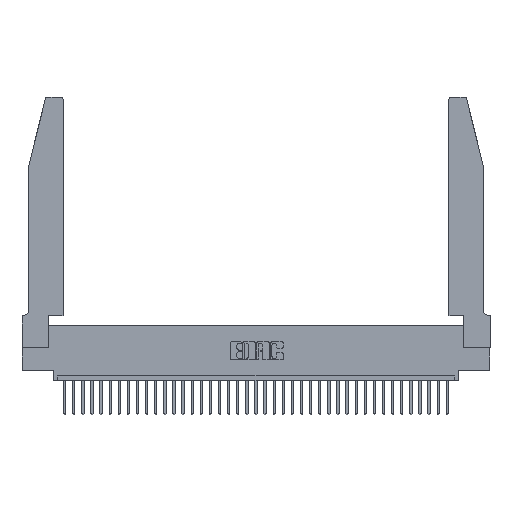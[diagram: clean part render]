
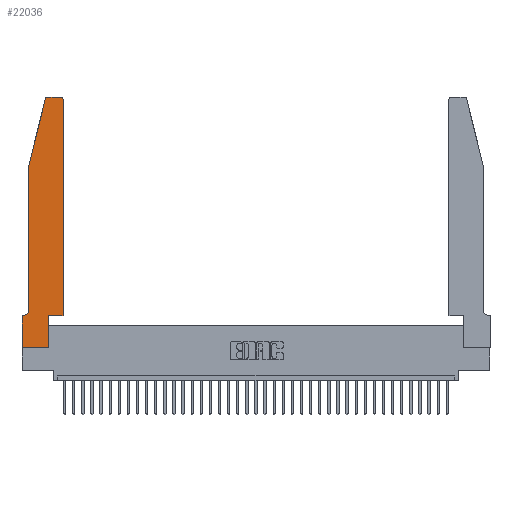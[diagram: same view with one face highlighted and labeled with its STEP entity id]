
A CAD part, top view. The second image highlights one B-rep face of the part: STEP entity #22036.
In plain terms, the highlighted planar face has unit normal (0, 0, 1).
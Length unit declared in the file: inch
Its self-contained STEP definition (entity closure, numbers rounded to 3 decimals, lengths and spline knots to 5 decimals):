
#515 = EDGE_CURVE ( 'NONE', #30148, #27316, #31399, .T. ) ;
#525 = EDGE_CURVE ( 'NONE', #15190, #22995, #31805, .T. ) ;
#536 = DIRECTION ( 'NONE',  ( 0., 0., -1. ) ) ;
#739 = AXIS2_PLACEMENT_3D ( 'NONE', #6330, #9229, #6590 ) ;
#1643 = EDGE_CURVE ( 'NONE', #19819, #7447, #14745, .T. ) ;
#2044 = DIRECTION ( 'NONE',  ( 0., 0., 1. ) ) ;
#2127 = VERTEX_POINT ( 'NONE', #19184 ) ;
#2597 = DIRECTION ( 'NONE',  ( 0., 0., 1. ) ) ;
#2716 = LINE ( 'NONE', #20206, #26402 ) ;
#3038 = DIRECTION ( 'NONE',  ( 0., 1., 0. ) ) ;
#3045 = LINE ( 'NONE', #9687, #5281 ) ;
#3090 = DIRECTION ( 'NONE',  ( -1., 0., 0. ) ) ;
#3216 = CARTESIAN_POINT ( 'NONE',  ( 0.4505, 2.72, 0.37 ) ) ;
#3639 = CARTESIAN_POINT ( 'NONE',  ( 0.0055, 0.35, 0.37 ) ) ;
#5055 = VERTEX_POINT ( 'NONE', #18728 ) ;
#5235 = AXIS2_PLACEMENT_3D ( 'NONE', #31842, #536, #20559 ) ;
#5281 = VECTOR ( 'NONE', #32691, 39.37008 ) ;
#5561 = CARTESIAN_POINT ( 'NONE',  ( 0.0755, 2., 0.37 ) ) ;
#5908 = VERTEX_POINT ( 'NONE', #22934 ) ;
#6234 = VECTOR ( 'NONE', #21673, 39.37008 ) ;
#6330 = CARTESIAN_POINT ( 'NONE',  ( 0.284, 2.72, 0.37 ) ) ;
#6590 = DIRECTION ( 'NONE',  ( 1., 0., 0. ) ) ;
#6735 = ORIENTED_EDGE ( 'NONE', *, *, #24252, .T. ) ;
#7035 = VECTOR ( 'NONE', #9014, 39.37008 ) ;
#7376 = ORIENTED_EDGE ( 'NONE', *, *, #33072, .T. ) ;
#7447 = VERTEX_POINT ( 'NONE', #3216 ) ;
#8647 = ORIENTED_EDGE ( 'NONE', *, *, #1643, .T. ) ;
#8999 = EDGE_CURVE ( 'NONE', #5908, #2127, #3045, .T. ) ;
#9014 = DIRECTION ( 'NONE',  ( 1., 0., 0. ) ) ;
#9229 = DIRECTION ( 'NONE',  ( 0., 0., 1. ) ) ;
#9687 = CARTESIAN_POINT ( 'NONE',  ( 0.0755, 2., 0.37 ) ) ;
#10422 = LINE ( 'NONE', #26447, #26007 ) ;
#11716 = EDGE_CURVE ( 'NONE', #7447, #5055, #19013, .T. ) ;
#12728 = AXIS2_PLACEMENT_3D ( 'NONE', #13175, #2044, #33209 ) ;
#13175 = CARTESIAN_POINT ( 'NONE',  ( 0., 0.35, 0.37 ) ) ;
#13645 = CARTESIAN_POINT ( 'NONE',  ( 0.4505, 0.35, 0.37 ) ) ;
#13721 = CARTESIAN_POINT ( 'NONE',  ( 0.4205, 2.72, 0.37 ) ) ;
#14286 = LINE ( 'NONE', #33466, #6234 ) ;
#14745 = LINE ( 'NONE', #13645, #28654 ) ;
#15190 = VERTEX_POINT ( 'NONE', #28389 ) ;
#15390 = VERTEX_POINT ( 'NONE', #33857 ) ;
#15525 = EDGE_CURVE ( 'NONE', #22995, #19819, #18051, .T. ) ;
#16125 = EDGE_LOOP ( 'NONE', ( #36950, #6735, #24460, #32511, #26265, #20859, #7376, #35809, #26120, #36816, #8647, #25574 ) ) ;
#16500 = EDGE_CURVE ( 'NONE', #27316, #15390, #10422, .T. ) ;
#17860 = VECTOR ( 'NONE', #34121, 39.37008 ) ;
#18051 = LINE ( 'NONE', #32734, #23875 ) ;
#18728 = CARTESIAN_POINT ( 'NONE',  ( 0.4205, 2.75, 0.37 ) ) ;
#18945 = EDGE_CURVE ( 'NONE', #28725, #15190, #23557, .T. ) ;
#19013 = CIRCLE ( 'NONE', #28277, 0.03 ) ;
#19156 = PLANE ( 'NONE',  #12728 ) ;
#19184 = CARTESIAN_POINT ( 'NONE',  ( 0.0755, 2., 0.37 ) ) ;
#19740 = VECTOR ( 'NONE', #3038, 39.37008 ) ;
#19819 = VERTEX_POINT ( 'NONE', #21456 ) ;
#20206 = CARTESIAN_POINT ( 'NONE',  ( 0.2605, 2.75, 0.37 ) ) ;
#20540 = DIRECTION ( 'NONE',  ( -1., 0., 0. ) ) ;
#20559 = DIRECTION ( 'NONE',  ( -1., 0., 0. ) ) ;
#20859 = ORIENTED_EDGE ( 'NONE', *, *, #16500, .T. ) ;
#21456 = CARTESIAN_POINT ( 'NONE',  ( 0.4505, 0.35, 0.37 ) ) ;
#21673 = DIRECTION ( 'NONE',  ( 0., -1., 0. ) ) ;
#22036 = ADVANCED_FACE ( 'NONE', ( #24678 ), #19156, .T. ) ;
#22313 = CIRCLE ( 'NONE', #739, 0.03 ) ;
#22330 = EDGE_CURVE ( 'NONE', #5055, #28479, #2716, .T. ) ;
#22761 = EDGE_CURVE ( 'NONE', #2127, #30148, #25500, .T. ) ;
#22934 = CARTESIAN_POINT ( 'NONE',  ( 0.25487, 2.72718, 0.37 ) ) ;
#22995 = VERTEX_POINT ( 'NONE', #35507 ) ;
#23557 = LINE ( 'NONE', #37129, #7035 ) ;
#23843 = CARTESIAN_POINT ( 'NONE',  ( 0.0755, 0.42, 0.37 ) ) ;
#23875 = VECTOR ( 'NONE', #32466, 39.37008 ) ;
#24252 = EDGE_CURVE ( 'NONE', #28479, #5908, #22313, .T. ) ;
#24460 = ORIENTED_EDGE ( 'NONE', *, *, #8999, .T. ) ;
#24678 = FACE_OUTER_BOUND ( 'NONE', #16125, .T. ) ;
#25222 = DIRECTION ( 'NONE',  ( 1., 0., 0. ) ) ;
#25500 = LINE ( 'NONE', #5561, #17860 ) ;
#25509 = CARTESIAN_POINT ( 'NONE',  ( 0., 0., 0.37 ) ) ;
#25574 = ORIENTED_EDGE ( 'NONE', *, *, #11716, .T. ) ;
#26007 = VECTOR ( 'NONE', #20540, 39.37008 ) ;
#26120 = ORIENTED_EDGE ( 'NONE', *, *, #525, .T. ) ;
#26265 = ORIENTED_EDGE ( 'NONE', *, *, #515, .T. ) ;
#26402 = VECTOR ( 'NONE', #3090, 39.37008 ) ;
#26447 = CARTESIAN_POINT ( 'NONE',  ( 0.0755, 0.35, 0.37 ) ) ;
#26752 = CARTESIAN_POINT ( 'NONE',  ( 0.284, 2.75, 0.37 ) ) ;
#27316 = VERTEX_POINT ( 'NONE', #3639 ) ;
#28277 = AXIS2_PLACEMENT_3D ( 'NONE', #13721, #2597, #25222 ) ;
#28389 = CARTESIAN_POINT ( 'NONE',  ( 0.2865, 0., 0.37 ) ) ;
#28479 = VERTEX_POINT ( 'NONE', #26752 ) ;
#28654 = VECTOR ( 'NONE', #33195, 39.37008 ) ;
#28725 = VERTEX_POINT ( 'NONE', #25509 ) ;
#30148 = VERTEX_POINT ( 'NONE', #23843 ) ;
#31399 = CIRCLE ( 'NONE', #5235, 0.07 ) ;
#31805 = LINE ( 'NONE', #35661, #19740 ) ;
#31842 = CARTESIAN_POINT ( 'NONE',  ( 0.0055, 0.42, 0.37 ) ) ;
#32466 = DIRECTION ( 'NONE',  ( 1., 0., 0. ) ) ;
#32511 = ORIENTED_EDGE ( 'NONE', *, *, #22761, .T. ) ;
#32691 = DIRECTION ( 'NONE',  ( -0.239, -0.971, 0. ) ) ;
#32734 = CARTESIAN_POINT ( 'NONE',  ( 0.4505, 0.35, 0.37 ) ) ;
#33072 = EDGE_CURVE ( 'NONE', #15390, #28725, #14286, .T. ) ;
#33195 = DIRECTION ( 'NONE',  ( 0., 1., 0. ) ) ;
#33209 = DIRECTION ( 'NONE',  ( 1., 0., 0. ) ) ;
#33466 = CARTESIAN_POINT ( 'NONE',  ( 0., 0., 0.37 ) ) ;
#33857 = CARTESIAN_POINT ( 'NONE',  ( 0., 0.35, 0.37 ) ) ;
#34121 = DIRECTION ( 'NONE',  ( 0., -1., 0. ) ) ;
#35507 = CARTESIAN_POINT ( 'NONE',  ( 0.2865, 0.35, 0.37 ) ) ;
#35661 = CARTESIAN_POINT ( 'NONE',  ( 0.2865, 0.35, 0.37 ) ) ;
#35809 = ORIENTED_EDGE ( 'NONE', *, *, #18945, .T. ) ;
#36816 = ORIENTED_EDGE ( 'NONE', *, *, #15525, .T. ) ;
#36950 = ORIENTED_EDGE ( 'NONE', *, *, #22330, .T. ) ;
#37129 = CARTESIAN_POINT ( 'NONE',  ( 0., 0., 0.37 ) ) ;
